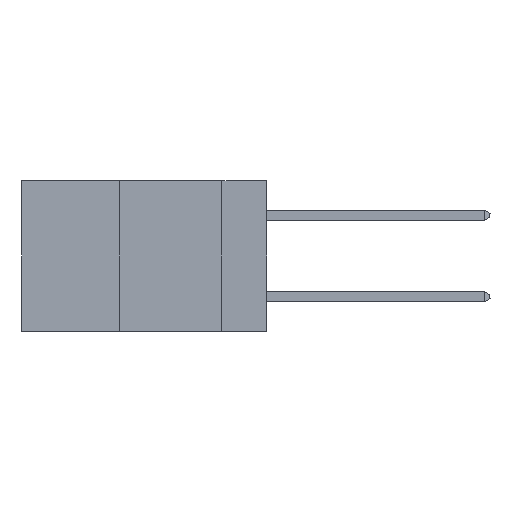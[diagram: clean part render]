
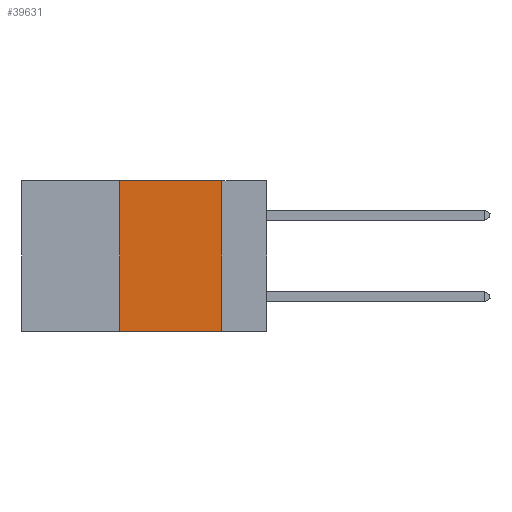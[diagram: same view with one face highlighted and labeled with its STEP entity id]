
A CAD part, left-side view. The second image highlights one B-rep face of the part: STEP entity #39631.
In plain terms, the highlighted planar face has unit normal (-1, 0, 0).
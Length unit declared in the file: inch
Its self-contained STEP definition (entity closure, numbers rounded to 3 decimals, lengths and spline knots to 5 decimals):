
#2273 = DIRECTION ( 'NONE',  ( 0., -1., 0. ) ) ;
#2806 = VERTEX_POINT ( 'NONE', #20034 ) ;
#3259 = CARTESIAN_POINT ( 'NONE',  ( 0., 0.6, 0. ) ) ;
#4563 = LINE ( 'NONE', #28570, #18325 ) ;
#4990 = ORIENTED_EDGE ( 'NONE', *, *, #7900, .T. ) ;
#5110 = EDGE_CURVE ( 'NONE', #11992, #2806, #29742, .T. ) ;
#7900 = EDGE_CURVE ( 'NONE', #36021, #2806, #18020, .T. ) ;
#9207 = DIRECTION ( 'NONE',  ( 0., 0., -1. ) ) ;
#10918 = LINE ( 'NONE', #3259, #17227 ) ;
#11992 = VERTEX_POINT ( 'NONE', #15486 ) ;
#12907 = PLANE ( 'NONE',  #33378 ) ;
#13067 = DIRECTION ( 'NONE',  ( 1., 0., 0. ) ) ;
#14895 = CARTESIAN_POINT ( 'NONE',  ( 0., 0.6, -0.37 ) ) ;
#15486 = CARTESIAN_POINT ( 'NONE',  ( 0., 0.11, 0. ) ) ;
#16340 = EDGE_CURVE ( 'NONE', #36021, #27127, #4563, .T. ) ;
#16546 = VECTOR ( 'NONE', #38080, 39.37008 ) ;
#17227 = VECTOR ( 'NONE', #2273, 39.37008 ) ;
#17788 = DIRECTION ( 'NONE',  ( 0., 0., 1. ) ) ;
#18020 = LINE ( 'NONE', #14895, #26056 ) ;
#18325 = VECTOR ( 'NONE', #17788, 39.37008 ) ;
#18399 = DIRECTION ( 'NONE',  ( 0., -1., 0. ) ) ;
#19805 = ORIENTED_EDGE ( 'NONE', *, *, #16340, .F. ) ;
#20034 = CARTESIAN_POINT ( 'NONE',  ( 0., 0.11, -0.37 ) ) ;
#21754 = CARTESIAN_POINT ( 'NONE',  ( 0., 0.36, 0. ) ) ;
#23476 = ORIENTED_EDGE ( 'NONE', *, *, #5110, .F. ) ;
#26056 = VECTOR ( 'NONE', #18399, 39.37008 ) ;
#26221 = CARTESIAN_POINT ( 'NONE',  ( 0., 0.36, -0.37 ) ) ;
#26813 = EDGE_LOOP ( 'NONE', ( #23476, #33193, #19805, #4990 ) ) ;
#27038 = CARTESIAN_POINT ( 'NONE',  ( 0., 0.11, 0. ) ) ;
#27127 = VERTEX_POINT ( 'NONE', #21754 ) ;
#28570 = CARTESIAN_POINT ( 'NONE',  ( 0., 0.36, 0. ) ) ;
#29742 = LINE ( 'NONE', #27038, #16546 ) ;
#30631 = EDGE_CURVE ( 'NONE', #27127, #11992, #10918, .T. ) ;
#33193 = ORIENTED_EDGE ( 'NONE', *, *, #30631, .F. ) ;
#33378 = AXIS2_PLACEMENT_3D ( 'NONE', #34874, #13067, #9207 ) ;
#34874 = CARTESIAN_POINT ( 'NONE',  ( 0., 0.6, 0. ) ) ;
#36021 = VERTEX_POINT ( 'NONE', #26221 ) ;
#38080 = DIRECTION ( 'NONE',  ( 0., 0., -1. ) ) ;
#39631 = ADVANCED_FACE ( 'NONE', ( #44423 ), #12907, .F. ) ;
#44423 = FACE_OUTER_BOUND ( 'NONE', #26813, .T. ) ;
